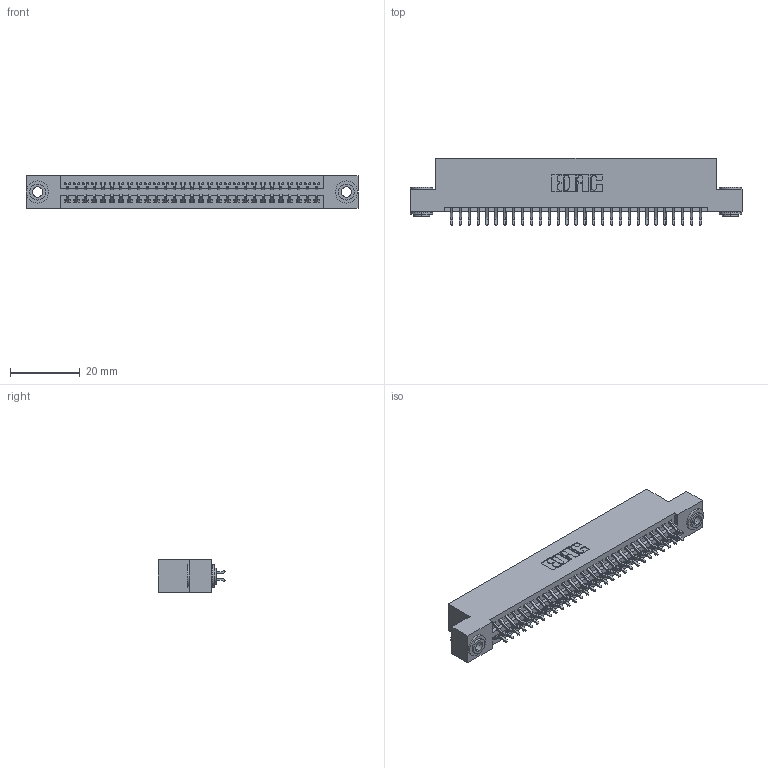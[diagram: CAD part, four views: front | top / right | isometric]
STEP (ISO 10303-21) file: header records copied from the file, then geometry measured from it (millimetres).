
FILE_DESCRIPTION (( 'STEP AP203' ), '1' );
FILE_NAME ('345-058-556-203.STEP', '2018-09-26T16:31:55', ( '' ), ( '' ), 'SwSTEP 2.0', 'SolidWorks 2016', '' );
FILE_SCHEMA (( 'CONFIG_CONTROL_DESIGN' ));
Length unit declared in the file: inch
Products named in the file (4): 345-250-002_345-250-002-102; 345-058-556-203; 345-292-001_556 Tail; 345 Part_Flush Mounting Lugs - 0.156 Dia-TH
Assembly tree (61 placements, depth 2):
  345-058-556-203
    345 Part_Flush Mounting Lugs - 0.156 Dia-TH
    345-292-001_556 Tail  x58
    345-250-002_345-250-002-102  x2
Bounding box: 94.87 x 19.24 x 9.4 mm (x, y, z)
Volume: 9112.1 mm3; surface area: 13371.6 mm2
Topology: 61 solids, 61 shells, 3412 faces, 10103 edges, 6654 vertices
Faces by surface type: plane 2236, cylinder 1168, cone 8
Entity records: 25374 total; most frequent: CARTESIAN_POINT 4255, ORIENTED_EDGE 4170, DIRECTION 3787, EDGE_CURVE 2085, LINE 1805, VECTOR 1805, VERTEX_POINT 1386, AXIS2_PLACEMENT_3D 991
